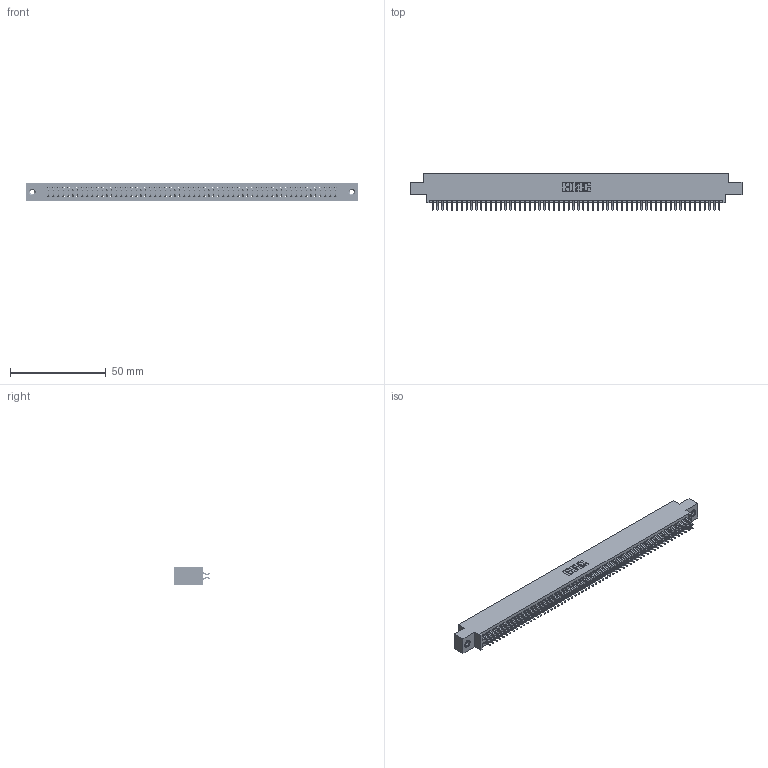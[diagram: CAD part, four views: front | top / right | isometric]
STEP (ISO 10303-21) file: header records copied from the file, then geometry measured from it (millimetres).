
FILE_DESCRIPTION (( 'STEP AP203' ), '1' );
FILE_NAME ('395-120-556-808.STEP', '2019-10-28T05:52:21', ( '' ), ( '' ), 'SwSTEP 2.0', 'SolidWorks 2016', '' );
FILE_SCHEMA (( 'CONFIG_CONTROL_DESIGN' ));
Length unit declared in the file: inch
Products named in the file (4): 345 Part_0.170 Offset - 0.156 Dia-TI; 345-292-001_556 Tail; 345-250-001_345-250-003-102; 395-120-556-808
Assembly tree (123 placements, depth 2):
  395-120-556-808
    345 Part_0.170 Offset - 0.156 Dia-TI
    345-292-001_556 Tail  x120
    345-250-001_345-250-003-102  x2
Bounding box: 173.61 x 19.24 x 9.4 mm (x, y, z)
Volume: 16907 mm3; surface area: 25391.8 mm2
Topology: 123 solids, 123 shells, 6910 faces, 20529 edges, 13518 vertices
Faces by surface type: plane 4556, cylinder 2338, cone 12, torus 4
Entity records: 46192 total; most frequent: CARTESIAN_POINT 7723, ORIENTED_EDGE 7638, DIRECTION 6801, EDGE_CURVE 3819, VECTOR 3419, LINE 3419, VERTEX_POINT 2540, AXIS2_PLACEMENT_3D 1691
